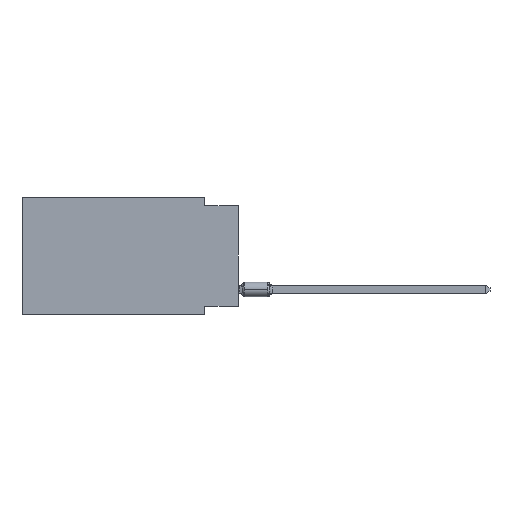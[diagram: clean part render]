
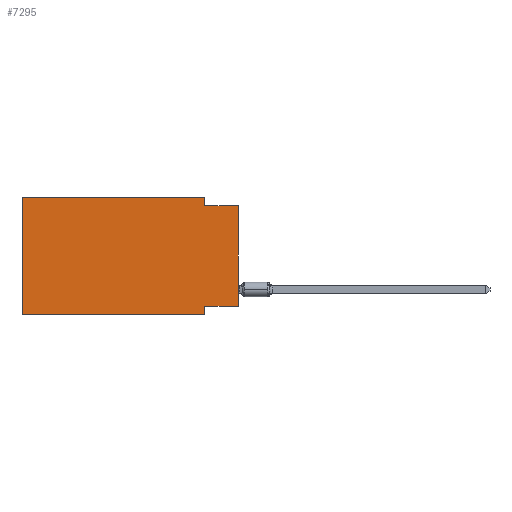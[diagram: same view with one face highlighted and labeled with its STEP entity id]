
A CAD part, left-side view. The second image highlights one B-rep face of the part: STEP entity #7295.
In plain terms, the highlighted planar face has unit normal (-1, 0, 0).
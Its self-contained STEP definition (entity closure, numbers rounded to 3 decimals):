
#76 = CARTESIAN_POINT ( 'NONE',  ( 0., 0., -0.635 ) ) ;
#163 = DIRECTION ( 'NONE',  ( 0., 0., -1. ) ) ;
#253 = CARTESIAN_POINT ( 'NONE',  ( 0., 2.54, -8.255 ) ) ;
#358 = ORIENTED_EDGE ( 'NONE', *, *, #12806, .F. ) ;
#401 = EDGE_CURVE ( 'NONE', #5324, #9801, #8440, .T. ) ;
#784 = ORIENTED_EDGE ( 'NONE', *, *, #2250, .T. ) ;
#1334 = ORIENTED_EDGE ( 'NONE', *, *, #9569, .F. ) ;
#2027 = CARTESIAN_POINT ( 'NONE',  ( 0., 2.54, -0.635 ) ) ;
#2040 = VECTOR ( 'NONE', #7417, 1000. ) ;
#2054 = ORIENTED_EDGE ( 'NONE', *, *, #401, .F. ) ;
#2120 = AXIS2_PLACEMENT_3D ( 'NONE', #7294, #5039, #2126 ) ;
#2126 = DIRECTION ( 'NONE',  ( 0., 0., -1. ) ) ;
#2250 = EDGE_CURVE ( 'NONE', #9320, #9801, #10994, .T. ) ;
#2418 = EDGE_CURVE ( 'NONE', #5432, #11000, #11662, .T. ) ;
#2637 = DIRECTION ( 'NONE',  ( 0., -1., 0. ) ) ;
#2872 = EDGE_LOOP ( 'NONE', ( #784, #2054, #358, #11005, #1334, #12650, #12387, #5320 ) ) ;
#3034 = VECTOR ( 'NONE', #11181, 1000. ) ;
#3575 = CARTESIAN_POINT ( 'NONE',  ( 0., 0., -8.255 ) ) ;
#3748 = CARTESIAN_POINT ( 'NONE',  ( 0., 2.54, 0. ) ) ;
#4330 = CARTESIAN_POINT ( 'NONE',  ( 0., 16.383, -8.89 ) ) ;
#4593 = LINE ( 'NONE', #10799, #9095 ) ;
#4610 = EDGE_CURVE ( 'NONE', #11702, #11000, #8848, .T. ) ;
#4618 = DIRECTION ( 'NONE',  ( 0., -1., 0. ) ) ;
#4983 = CARTESIAN_POINT ( 'NONE',  ( 0., 0., 0. ) ) ;
#5039 = DIRECTION ( 'NONE',  ( 1., 0., 0. ) ) ;
#5176 = CARTESIAN_POINT ( 'NONE',  ( 0., 16.383, 0. ) ) ;
#5320 = ORIENTED_EDGE ( 'NONE', *, *, #5401, .F. ) ;
#5324 = VERTEX_POINT ( 'NONE', #2027 ) ;
#5401 = EDGE_CURVE ( 'NONE', #9320, #5432, #7600, .T. ) ;
#5432 = VERTEX_POINT ( 'NONE', #253 ) ;
#6061 = LINE ( 'NONE', #5176, #3034 ) ;
#6213 = VECTOR ( 'NONE', #163, 1000. ) ;
#6972 = DIRECTION ( 'NONE',  ( 0., 0., 1. ) ) ;
#7294 = CARTESIAN_POINT ( 'NONE',  ( 0., 16.383, 0. ) ) ;
#7295 = ADVANCED_FACE ( 'NONE', ( #12267 ), #8388, .F. ) ;
#7388 = VERTEX_POINT ( 'NONE', #12675 ) ;
#7417 = DIRECTION ( 'NONE',  ( 0., -1., 0. ) ) ;
#7600 = LINE ( 'NONE', #3575, #9434 ) ;
#8016 = CARTESIAN_POINT ( 'NONE',  ( 0., 2.54, 0. ) ) ;
#8388 = PLANE ( 'NONE',  #2120 ) ;
#8440 = LINE ( 'NONE', #76, #2040 ) ;
#8762 = DIRECTION ( 'NONE',  ( 0., 1., 0. ) ) ;
#8848 = LINE ( 'NONE', #9804, #11062 ) ;
#8926 = CARTESIAN_POINT ( 'NONE',  ( 0., 0., -0.635 ) ) ;
#9095 = VECTOR ( 'NONE', #2637, 1000. ) ;
#9320 = VERTEX_POINT ( 'NONE', #9568 ) ;
#9434 = VECTOR ( 'NONE', #8762, 1000. ) ;
#9496 = VECTOR ( 'NONE', #6972, 1000. ) ;
#9568 = CARTESIAN_POINT ( 'NONE',  ( 0., 0., -8.255 ) ) ;
#9569 = EDGE_CURVE ( 'NONE', #11702, #7388, #6061, .T. ) ;
#9801 = VERTEX_POINT ( 'NONE', #8926 ) ;
#9804 = CARTESIAN_POINT ( 'NONE',  ( 0., 16.383, -8.89 ) ) ;
#9949 = LINE ( 'NONE', #3748, #12636 ) ;
#10565 = EDGE_CURVE ( 'NONE', #7388, #13206, #4593, .T. ) ;
#10651 = CARTESIAN_POINT ( 'NONE',  ( 0., 2.54, -8.89 ) ) ;
#10799 = CARTESIAN_POINT ( 'NONE',  ( 0., 16.383, 0. ) ) ;
#10994 = LINE ( 'NONE', #4983, #9496 ) ;
#11000 = VERTEX_POINT ( 'NONE', #12945 ) ;
#11005 = ORIENTED_EDGE ( 'NONE', *, *, #10565, .F. ) ;
#11062 = VECTOR ( 'NONE', #4618, 1000. ) ;
#11181 = DIRECTION ( 'NONE',  ( 0., 0., 1. ) ) ;
#11662 = LINE ( 'NONE', #10651, #6213 ) ;
#11702 = VERTEX_POINT ( 'NONE', #4330 ) ;
#12267 = FACE_OUTER_BOUND ( 'NONE', #2872, .T. ) ;
#12387 = ORIENTED_EDGE ( 'NONE', *, *, #2418, .F. ) ;
#12636 = VECTOR ( 'NONE', #13205, 1000. ) ;
#12650 = ORIENTED_EDGE ( 'NONE', *, *, #4610, .T. ) ;
#12675 = CARTESIAN_POINT ( 'NONE',  ( 0., 16.383, 0. ) ) ;
#12806 = EDGE_CURVE ( 'NONE', #13206, #5324, #9949, .T. ) ;
#12945 = CARTESIAN_POINT ( 'NONE',  ( 0., 2.54, -8.89 ) ) ;
#13205 = DIRECTION ( 'NONE',  ( 0., 0., -1. ) ) ;
#13206 = VERTEX_POINT ( 'NONE', #8016 ) ;
